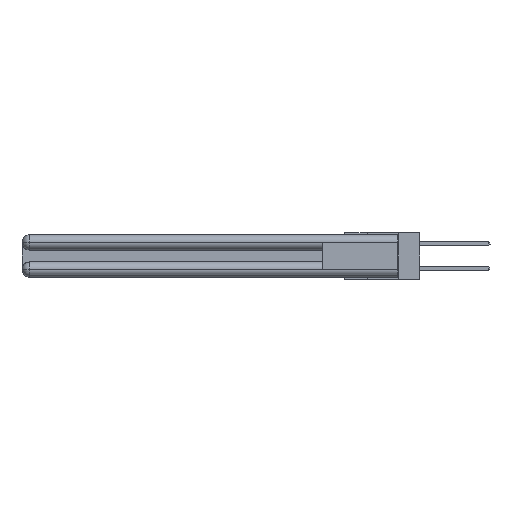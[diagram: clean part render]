
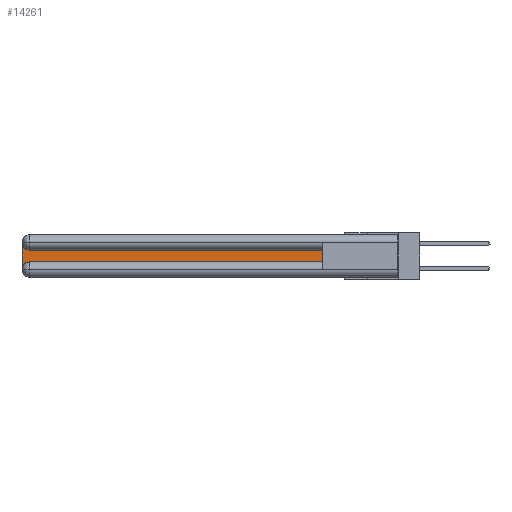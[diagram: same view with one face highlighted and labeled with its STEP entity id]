
A CAD part, left-side view. The second image highlights one B-rep face of the part: STEP entity #14261.
In plain terms, the highlighted planar face has unit normal (-1, 0, 0).
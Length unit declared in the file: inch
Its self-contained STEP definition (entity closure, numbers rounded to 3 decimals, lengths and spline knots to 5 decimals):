
#342 = AXIS2_PLACEMENT_3D ( 'NONE', #23584, #5520, #935 ) ;
#498 = DIRECTION ( 'NONE',  ( 1., 0., 0. ) ) ;
#629 = VECTOR ( 'NONE', #26540, 39.37008 ) ;
#935 = DIRECTION ( 'NONE',  ( 0., 0., -1. ) ) ;
#1582 = VECTOR ( 'NONE', #19654, 39.37008 ) ;
#1703 = LINE ( 'NONE', #5964, #18856 ) ;
#1718 = VERTEX_POINT ( 'NONE', #9364 ) ;
#2002 = CARTESIAN_POINT ( 'NONE',  ( 0.075, 0.6, -0.2175 ) ) ;
#2236 = VECTOR ( 'NONE', #8834, 39.37008 ) ;
#2509 = CARTESIAN_POINT ( 'NONE',  ( 0.075, 0.6, -0.1225 ) ) ;
#3359 = DIRECTION ( 'NONE',  ( 1., 0., 0. ) ) ;
#3870 = AXIS2_PLACEMENT_3D ( 'NONE', #21828, #3359, #26375 ) ;
#4431 = EDGE_CURVE ( 'NONE', #11259, #9001, #7568, .T. ) ;
#5022 = ORIENTED_EDGE ( 'NONE', *, *, #4431, .T. ) ;
#5520 = DIRECTION ( 'NONE',  ( 1., 0., 0. ) ) ;
#5964 = CARTESIAN_POINT ( 'NONE',  ( 0.075, 0.6, -0.2175 ) ) ;
#6081 = ORIENTED_EDGE ( 'NONE', *, *, #15095, .T. ) ;
#7568 = LINE ( 'NONE', #26339, #629 ) ;
#8442 = LINE ( 'NONE', #2002, #2236 ) ;
#8834 = DIRECTION ( 'NONE',  ( 0., -1., 0. ) ) ;
#8996 = CIRCLE ( 'NONE', #14608, 0.06 ) ;
#9001 = VERTEX_POINT ( 'NONE', #27456 ) ;
#9364 = CARTESIAN_POINT ( 'NONE',  ( 0.075, 2.94, -0.2175 ) ) ;
#10181 = EDGE_CURVE ( 'NONE', #1718, #11279, #8442, .T. ) ;
#11186 = ORIENTED_EDGE ( 'NONE', *, *, #18521, .T. ) ;
#11259 = VERTEX_POINT ( 'NONE', #2509 ) ;
#11279 = VERTEX_POINT ( 'NONE', #27133 ) ;
#12018 = CARTESIAN_POINT ( 'NONE',  ( 0.075, 2.94, -0.2775 ) ) ;
#12790 = EDGE_CURVE ( 'NONE', #30102, #1718, #8996, .T. ) ;
#13672 = EDGE_CURVE ( 'NONE', #9001, #23337, #20506, .T. ) ;
#13918 = CARTESIAN_POINT ( 'NONE',  ( 0.075, 3., -0.2775 ) ) ;
#14261 = ADVANCED_FACE ( 'NONE', ( #18416 ), #21729, .F. ) ;
#14340 = ORIENTED_EDGE ( 'NONE', *, *, #12790, .T. ) ;
#14608 = AXIS2_PLACEMENT_3D ( 'NONE', #12018, #498, #16815 ) ;
#15095 = EDGE_CURVE ( 'NONE', #23337, #30102, #27834, .T. ) ;
#16815 = DIRECTION ( 'NONE',  ( 0., 0., -1. ) ) ;
#17329 = ORIENTED_EDGE ( 'NONE', *, *, #10181, .T. ) ;
#18416 = FACE_OUTER_BOUND ( 'NONE', #19585, .T. ) ;
#18521 = EDGE_CURVE ( 'NONE', #11279, #11259, #1703, .T. ) ;
#18856 = VECTOR ( 'NONE', #29915, 39.37008 ) ;
#19585 = EDGE_LOOP ( 'NONE', ( #5022, #27153, #6081, #14340, #17329, #11186 ) ) ;
#19654 = DIRECTION ( 'NONE',  ( 0., 0., -1. ) ) ;
#20506 = CIRCLE ( 'NONE', #342, 0.06 ) ;
#21729 = PLANE ( 'NONE',  #3870 ) ;
#21828 = CARTESIAN_POINT ( 'NONE',  ( 0.075, 3., -0.1225 ) ) ;
#23337 = VERTEX_POINT ( 'NONE', #28946 ) ;
#23584 = CARTESIAN_POINT ( 'NONE',  ( 0.075, 2.94, -0.0625 ) ) ;
#26339 = CARTESIAN_POINT ( 'NONE',  ( 0.075, 0.6, -0.1225 ) ) ;
#26354 = CARTESIAN_POINT ( 'NONE',  ( 0.075, 3., -0.2175 ) ) ;
#26375 = DIRECTION ( 'NONE',  ( 0., 0., -1. ) ) ;
#26540 = DIRECTION ( 'NONE',  ( 0., 1., 0. ) ) ;
#27133 = CARTESIAN_POINT ( 'NONE',  ( 0.075, 0.6, -0.2175 ) ) ;
#27153 = ORIENTED_EDGE ( 'NONE', *, *, #13672, .T. ) ;
#27456 = CARTESIAN_POINT ( 'NONE',  ( 0.075, 2.94, -0.1225 ) ) ;
#27834 = LINE ( 'NONE', #26354, #1582 ) ;
#28946 = CARTESIAN_POINT ( 'NONE',  ( 0.075, 3., -0.0625 ) ) ;
#29915 = DIRECTION ( 'NONE',  ( 0., 0., 1. ) ) ;
#30102 = VERTEX_POINT ( 'NONE', #13918 ) ;
